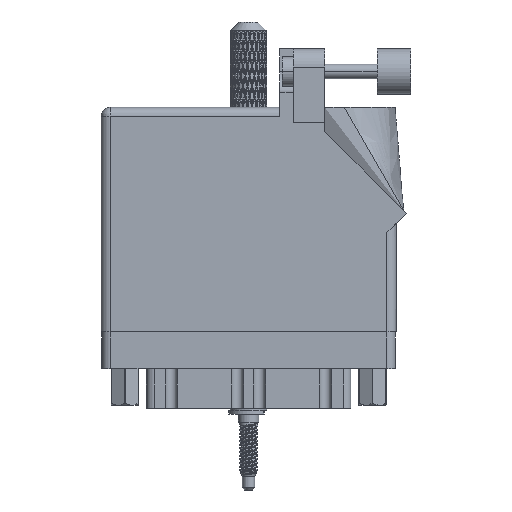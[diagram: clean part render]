
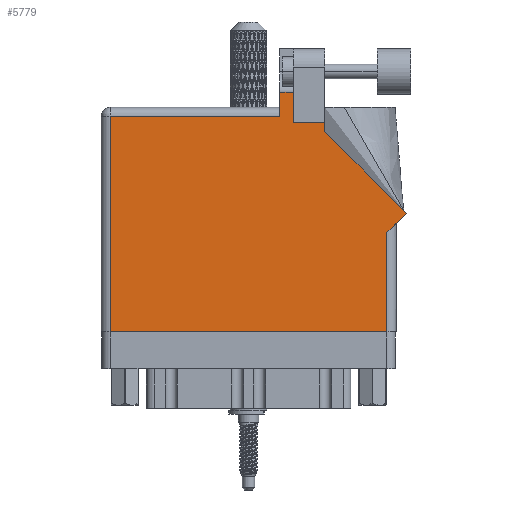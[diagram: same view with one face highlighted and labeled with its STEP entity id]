
A CAD part, front view. The second image highlights one B-rep face of the part: STEP entity #5779.
In plain terms, the highlighted face is planar.
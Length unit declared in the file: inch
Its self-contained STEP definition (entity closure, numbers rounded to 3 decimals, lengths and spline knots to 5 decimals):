
#1201 = CARTESIAN_POINT ( 'NONE',  ( 1.524, 1.36442, 0. ) ) ;
#2256 = CARTESIAN_POINT ( 'NONE',  ( 0., 0., 0. ) ) ;
#3399 = DIRECTION ( 'NONE',  ( 1., 0., 0. ) ) ;
#3467 = VECTOR ( 'NONE', #101034, 39.37008 ) ;
#3579 = CARTESIAN_POINT ( 'NONE',  ( 1.217, 1.6315, 0. ) ) ;
#3734 = CARTESIAN_POINT ( 'NONE',  ( 0.062, 0., 0. ) ) ;
#4765 = VECTOR ( 'NONE', #87232, 39.37008 ) ;
#5779 = ADVANCED_FACE ( 'NONE', ( #71126 ), #80282, .F. ) ;
#6247 = CARTESIAN_POINT ( 'NONE',  ( 2.08071, 0.80771, 0. ) ) ;
#8225 = VECTOR ( 'NONE', #58991, 39.37008 ) ;
#8426 = CARTESIAN_POINT ( 'NONE',  ( 1.311, 1.43, 0. ) ) ;
#9809 = ORIENTED_EDGE ( 'NONE', *, *, #77292, .T. ) ;
#11491 = VECTOR ( 'NONE', #18218, 39.37008 ) ;
#14273 = EDGE_CURVE ( 'NONE', #28803, #58178, #67101, .T. ) ;
#14567 = EDGE_CURVE ( 'NONE', #58307, #56186, #27993, .T. ) ;
#15040 = VERTEX_POINT ( 'NONE', #51028 ) ;
#16109 = VERTEX_POINT ( 'NONE', #78460 ) ;
#16352 = ORIENTED_EDGE ( 'NONE', *, *, #50774, .T. ) ;
#18218 = DIRECTION ( 'NONE',  ( 0., 1., 0. ) ) ;
#19194 = LINE ( 'NONE', #29524, #23226 ) ;
#20348 = ORIENTED_EDGE ( 'NONE', *, *, #46283, .T. ) ;
#22264 = CARTESIAN_POINT ( 'NONE',  ( 1.311, 1.43, 0. ) ) ;
#23226 = VECTOR ( 'NONE', #28370, 39.37008 ) ;
#24795 = LINE ( 'NONE', #78158, #72629 ) ;
#26883 = AXIS2_PLACEMENT_3D ( 'NONE', #88885, #107773, #64164 ) ;
#27222 = VECTOR ( 'NONE', #70004, 39.37008 ) ;
#27993 = LINE ( 'NONE', #43540, #37435 ) ;
#28083 = CARTESIAN_POINT ( 'NONE',  ( 1.217, 1.468, 0. ) ) ;
#28370 = DIRECTION ( 'NONE',  ( 0.707, 0.707, 0. ) ) ;
#28803 = VERTEX_POINT ( 'NONE', #3579 ) ;
#29042 = VERTEX_POINT ( 'NONE', #1201 ) ;
#29112 = ORIENTED_EDGE ( 'NONE', *, *, #109427, .T. ) ;
#29524 = CARTESIAN_POINT ( 'NONE',  ( 2.01, 0.737, 0. ) ) ;
#31559 = LINE ( 'NONE', #38482, #3467 ) ;
#33508 = EDGE_CURVE ( 'NONE', #80369, #58307, #72367, .T. ) ;
#34046 = CARTESIAN_POINT ( 'NONE',  ( 1.948, 0., 0. ) ) ;
#37435 = VECTOR ( 'NONE', #78588, 39.37008 ) ;
#38258 = ORIENTED_EDGE ( 'NONE', *, *, #14567, .T. ) ;
#38482 = CARTESIAN_POINT ( 'NONE',  ( 0.062, 0., 0. ) ) ;
#40700 = CARTESIAN_POINT ( 'NONE',  ( 1.217, 1.53, 0. ) ) ;
#42014 = LINE ( 'NONE', #100752, #103831 ) ;
#42636 = ORIENTED_EDGE ( 'NONE', *, *, #111683, .T. ) ;
#43540 = CARTESIAN_POINT ( 'NONE',  ( 1.948, 0.737, 0. ) ) ;
#43589 = LINE ( 'NONE', #6247, #27222 ) ;
#45539 = VERTEX_POINT ( 'NONE', #62344 ) ;
#46283 = EDGE_CURVE ( 'NONE', #73019, #16109, #95731, .T. ) ;
#48656 = LINE ( 'NONE', #57273, #8225 ) ;
#48713 = ORIENTED_EDGE ( 'NONE', *, *, #33508, .T. ) ;
#48723 = VERTEX_POINT ( 'NONE', #98848 ) ;
#49306 = DIRECTION ( 'NONE',  ( 0., -1., 0. ) ) ;
#50774 = EDGE_CURVE ( 'NONE', #48723, #73019, #48656, .T. ) ;
#51028 = CARTESIAN_POINT ( 'NONE',  ( 0.062, 1.468, 0. ) ) ;
#52187 = CARTESIAN_POINT ( 'NONE',  ( 0., 1.468, 0. ) ) ;
#56186 = VERTEX_POINT ( 'NONE', #71224 ) ;
#57273 = CARTESIAN_POINT ( 'NONE',  ( 1.524, 1.43, 0. ) ) ;
#58178 = VERTEX_POINT ( 'NONE', #28083 ) ;
#58307 = VERTEX_POINT ( 'NONE', #34046 ) ;
#58991 = DIRECTION ( 'NONE',  ( -1., 0., 0. ) ) ;
#62344 = CARTESIAN_POINT ( 'NONE',  ( 2.08071, 0.80771, 0. ) ) ;
#63033 = LINE ( 'NONE', #52187, #4765 ) ;
#64164 = DIRECTION ( 'NONE',  ( -1., 0., 0. ) ) ;
#67101 = LINE ( 'NONE', #40700, #86974 ) ;
#70004 = DIRECTION ( 'NONE',  ( -0.707, 0.707, 0. ) ) ;
#70209 = ORIENTED_EDGE ( 'NONE', *, *, #14273, .T. ) ;
#71126 = FACE_OUTER_BOUND ( 'NONE', #111333, .T. ) ;
#71224 = CARTESIAN_POINT ( 'NONE',  ( 1.948, 0.675, 0. ) ) ;
#71769 = ORIENTED_EDGE ( 'NONE', *, *, #104271, .T. ) ;
#72367 = LINE ( 'NONE', #2256, #109760 ) ;
#72629 = VECTOR ( 'NONE', #94839, 39.37008 ) ;
#73019 = VERTEX_POINT ( 'NONE', #22264 ) ;
#77041 = DIRECTION ( 'NONE',  ( -1., 0., 0. ) ) ;
#77292 = EDGE_CURVE ( 'NONE', #58178, #15040, #63033, .T. ) ;
#78158 = CARTESIAN_POINT ( 'NONE',  ( 1.524, 1.36442, 0. ) ) ;
#78460 = CARTESIAN_POINT ( 'NONE',  ( 1.311, 1.6315, 0. ) ) ;
#78588 = DIRECTION ( 'NONE',  ( 0., 1., 0. ) ) ;
#80282 = PLANE ( 'NONE',  #26883 ) ;
#80369 = VERTEX_POINT ( 'NONE', #3734 ) ;
#83664 = EDGE_CURVE ( 'NONE', #56186, #45539, #19194, .T. ) ;
#86974 = VECTOR ( 'NONE', #49306, 39.37008 ) ;
#87232 = DIRECTION ( 'NONE',  ( -1., 0., 0. ) ) ;
#88885 = CARTESIAN_POINT ( 'NONE',  ( 0., 1.53, 0. ) ) ;
#92177 = ORIENTED_EDGE ( 'NONE', *, *, #83664, .T. ) ;
#94839 = DIRECTION ( 'NONE',  ( 0., 1., 0. ) ) ;
#95731 = LINE ( 'NONE', #8426, #11491 ) ;
#97497 = ORIENTED_EDGE ( 'NONE', *, *, #105071, .T. ) ;
#98848 = CARTESIAN_POINT ( 'NONE',  ( 1.524, 1.43, 0. ) ) ;
#100752 = CARTESIAN_POINT ( 'NONE',  ( 1.64177, 1.6315, 0. ) ) ;
#101034 = DIRECTION ( 'NONE',  ( 0., -1., 0. ) ) ;
#103831 = VECTOR ( 'NONE', #77041, 39.37008 ) ;
#104271 = EDGE_CURVE ( 'NONE', #29042, #48723, #24795, .T. ) ;
#105071 = EDGE_CURVE ( 'NONE', #16109, #28803, #42014, .T. ) ;
#107773 = DIRECTION ( 'NONE',  ( 0., 0., -1. ) ) ;
#109427 = EDGE_CURVE ( 'NONE', #45539, #29042, #43589, .T. ) ;
#109760 = VECTOR ( 'NONE', #3399, 39.37008 ) ;
#111333 = EDGE_LOOP ( 'NONE', ( #20348, #97497, #70209, #9809, #42636, #48713, #38258, #92177, #29112, #71769, #16352 ) ) ;
#111683 = EDGE_CURVE ( 'NONE', #15040, #80369, #31559, .T. ) ;
